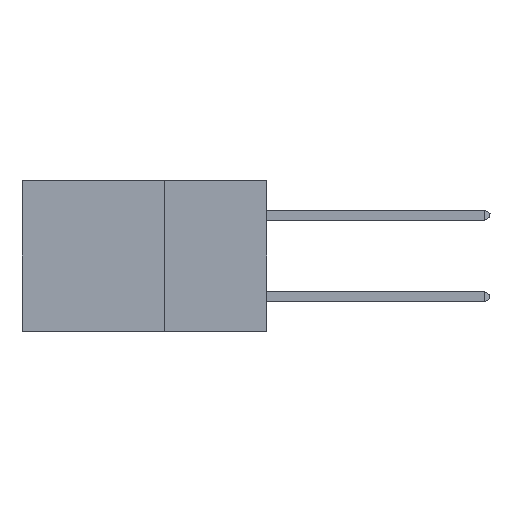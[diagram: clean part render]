
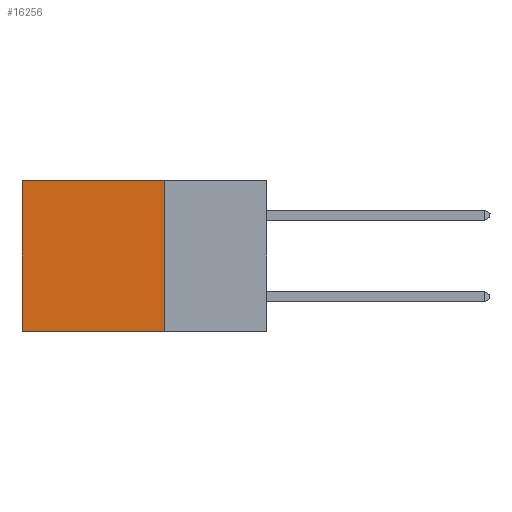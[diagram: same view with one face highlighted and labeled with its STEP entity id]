
A CAD part, left-side view. The second image highlights one B-rep face of the part: STEP entity #16256.
In plain terms, the highlighted planar face has unit normal (-1, 0, 0).
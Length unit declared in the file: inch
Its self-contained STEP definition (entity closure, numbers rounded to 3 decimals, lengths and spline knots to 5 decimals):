
#416 = LINE ( 'NONE', #4943, #21204 ) ;
#593 = CARTESIAN_POINT ( 'NONE',  ( 0.2875, 0.6, -0.37 ) ) ;
#2059 = CARTESIAN_POINT ( 'NONE',  ( 0.2875, 0.6, 0. ) ) ;
#2430 = ORIENTED_EDGE ( 'NONE', *, *, #9751, .T. ) ;
#3133 = ORIENTED_EDGE ( 'NONE', *, *, #19073, .F. ) ;
#3405 = VECTOR ( 'NONE', #7125, 39.37008 ) ;
#4713 = CARTESIAN_POINT ( 'NONE',  ( 0.2875, 0.25, -0.37 ) ) ;
#4891 = CARTESIAN_POINT ( 'NONE',  ( 0.2875, 0.25, -0.37 ) ) ;
#4943 = CARTESIAN_POINT ( 'NONE',  ( 0.2875, 0.25, 0. ) ) ;
#4991 = AXIS2_PLACEMENT_3D ( 'NONE', #21446, #14971, #18241 ) ;
#5114 = CARTESIAN_POINT ( 'NONE',  ( 0.2875, 0.25, 0. ) ) ;
#6186 = DIRECTION ( 'NONE',  ( 0., 0., -1. ) ) ;
#7125 = DIRECTION ( 'NONE',  ( 0., 0., -1. ) ) ;
#7192 = VERTEX_POINT ( 'NONE', #5114 ) ;
#7528 = LINE ( 'NONE', #19478, #21139 ) ;
#7594 = ORIENTED_EDGE ( 'NONE', *, *, #17888, .F. ) ;
#8363 = DIRECTION ( 'NONE',  ( 0., 1., 0. ) ) ;
#9403 = CARTESIAN_POINT ( 'NONE',  ( 0.2875, 0.6, 0. ) ) ;
#9751 = EDGE_CURVE ( 'NONE', #7192, #11532, #416, .T. ) ;
#10041 = VERTEX_POINT ( 'NONE', #4891 ) ;
#10088 = VERTEX_POINT ( 'NONE', #593 ) ;
#11532 = VERTEX_POINT ( 'NONE', #9403 ) ;
#13518 = EDGE_LOOP ( 'NONE', ( #17500, #3133, #7594, #2430 ) ) ;
#13596 = LINE ( 'NONE', #2059, #3405 ) ;
#14971 = DIRECTION ( 'NONE',  ( 1., 0., 0. ) ) ;
#16256 = ADVANCED_FACE ( 'NONE', ( #20014 ), #18039, .F. ) ;
#17500 = ORIENTED_EDGE ( 'NONE', *, *, #20085, .T. ) ;
#17888 = EDGE_CURVE ( 'NONE', #7192, #10041, #7528, .T. ) ;
#18039 = PLANE ( 'NONE',  #4991 ) ;
#18241 = DIRECTION ( 'NONE',  ( 0., 0., -1. ) ) ;
#19073 = EDGE_CURVE ( 'NONE', #10041, #10088, #21489, .T. ) ;
#19478 = CARTESIAN_POINT ( 'NONE',  ( 0.2875, 0.25, 0. ) ) ;
#19952 = DIRECTION ( 'NONE',  ( 0., 1., 0. ) ) ;
#20014 = FACE_OUTER_BOUND ( 'NONE', #13518, .T. ) ;
#20085 = EDGE_CURVE ( 'NONE', #11532, #10088, #13596, .T. ) ;
#20811 = VECTOR ( 'NONE', #19952, 39.37008 ) ;
#21139 = VECTOR ( 'NONE', #6186, 39.37008 ) ;
#21204 = VECTOR ( 'NONE', #8363, 39.37008 ) ;
#21446 = CARTESIAN_POINT ( 'NONE',  ( 0.2875, 0.25, 0. ) ) ;
#21489 = LINE ( 'NONE', #4713, #20811 ) ;
